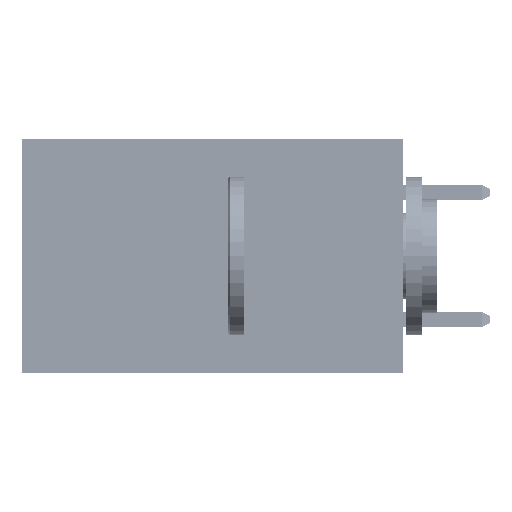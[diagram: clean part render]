
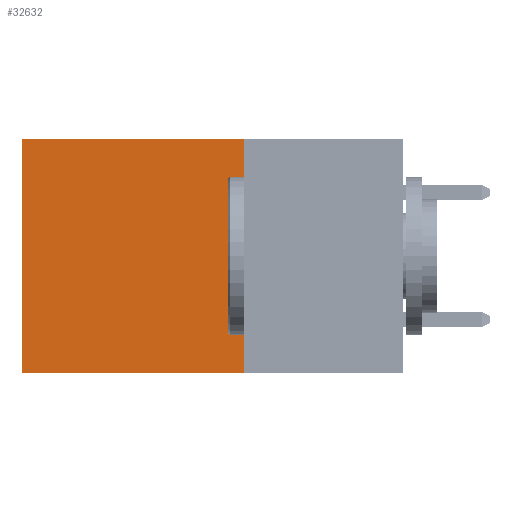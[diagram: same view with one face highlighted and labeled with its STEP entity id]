
A CAD part, left-side view. The second image highlights one B-rep face of the part: STEP entity #32632.
In plain terms, the highlighted planar face has unit normal (-1, 0, 0).
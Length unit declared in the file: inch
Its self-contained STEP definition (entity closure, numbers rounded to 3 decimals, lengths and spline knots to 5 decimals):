
#2707 = CARTESIAN_POINT ( 'NONE',  ( 0.2875, 0.6, -0.37 ) ) ;
#3137 = VERTEX_POINT ( 'NONE', #2707 ) ;
#4332 = CARTESIAN_POINT ( 'NONE',  ( 0.2875, 0.25, -0.37 ) ) ;
#7389 = VERTEX_POINT ( 'NONE', #40331 ) ;
#8863 = CARTESIAN_POINT ( 'NONE',  ( 0.2875, 0.25, 0. ) ) ;
#9505 = EDGE_CURVE ( 'NONE', #7389, #3137, #26461, .T. ) ;
#11481 = EDGE_LOOP ( 'NONE', ( #27598, #20162, #42420, #17299 ) ) ;
#14476 = VECTOR ( 'NONE', #36791, 39.37008 ) ;
#14664 = CARTESIAN_POINT ( 'NONE',  ( 0.2875, 0.6, 0. ) ) ;
#16245 = DIRECTION ( 'NONE',  ( 0., 1., 0. ) ) ;
#17299 = ORIENTED_EDGE ( 'NONE', *, *, #28829, .T. ) ;
#18024 = EDGE_CURVE ( 'NONE', #41543, #25094, #32142, .T. ) ;
#18941 = DIRECTION ( 'NONE',  ( 1., 0., 0. ) ) ;
#20162 = ORIENTED_EDGE ( 'NONE', *, *, #40350, .F. ) ;
#25094 = VERTEX_POINT ( 'NONE', #29313 ) ;
#26461 = LINE ( 'NONE', #14664, #14476 ) ;
#27598 = ORIENTED_EDGE ( 'NONE', *, *, #9505, .T. ) ;
#28829 = EDGE_CURVE ( 'NONE', #41543, #7389, #37131, .T. ) ;
#29313 = CARTESIAN_POINT ( 'NONE',  ( 0.2875, 0.25, -0.37 ) ) ;
#29880 = DIRECTION ( 'NONE',  ( 0., 1., 0. ) ) ;
#32142 = LINE ( 'NONE', #8863, #41364 ) ;
#32632 = ADVANCED_FACE ( 'NONE', ( #37975 ), #40765, .F. ) ;
#33135 = LINE ( 'NONE', #4332, #34270 ) ;
#33425 = CARTESIAN_POINT ( 'NONE',  ( 0.2875, 0.25, 0. ) ) ;
#34270 = VECTOR ( 'NONE', #29880, 39.37008 ) ;
#35337 = CARTESIAN_POINT ( 'NONE',  ( 0.2875, 0.25, 0. ) ) ;
#36791 = DIRECTION ( 'NONE',  ( 0., 0., -1. ) ) ;
#37131 = LINE ( 'NONE', #41747, #45709 ) ;
#37881 = DIRECTION ( 'NONE',  ( 0., 0., -1. ) ) ;
#37975 = FACE_OUTER_BOUND ( 'NONE', #11481, .T. ) ;
#40331 = CARTESIAN_POINT ( 'NONE',  ( 0.2875, 0.6, 0. ) ) ;
#40350 = EDGE_CURVE ( 'NONE', #25094, #3137, #33135, .T. ) ;
#40765 = PLANE ( 'NONE',  #41177 ) ;
#41177 = AXIS2_PLACEMENT_3D ( 'NONE', #33425, #18941, #44443 ) ;
#41364 = VECTOR ( 'NONE', #37881, 39.37008 ) ;
#41543 = VERTEX_POINT ( 'NONE', #35337 ) ;
#41747 = CARTESIAN_POINT ( 'NONE',  ( 0.2875, 0.25, 0. ) ) ;
#42420 = ORIENTED_EDGE ( 'NONE', *, *, #18024, .F. ) ;
#44443 = DIRECTION ( 'NONE',  ( 0., 0., -1. ) ) ;
#45709 = VECTOR ( 'NONE', #16245, 39.37008 ) ;
